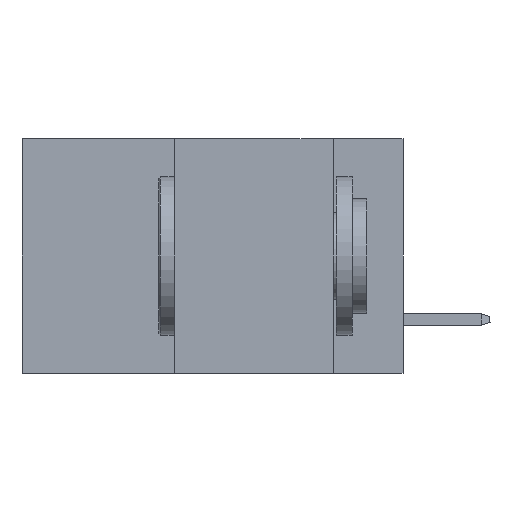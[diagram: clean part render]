
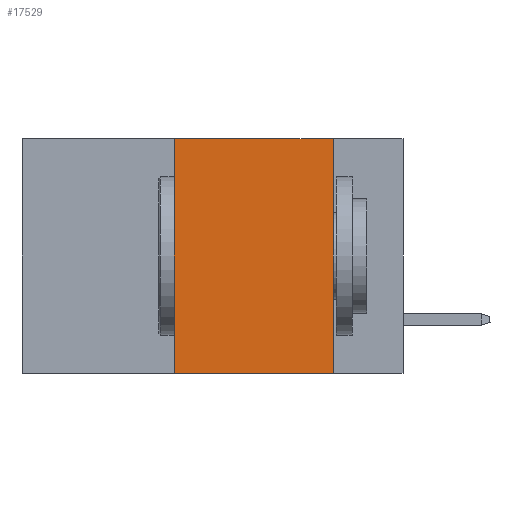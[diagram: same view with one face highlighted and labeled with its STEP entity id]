
A CAD part, left-side view. The second image highlights one B-rep face of the part: STEP entity #17529.
In plain terms, the highlighted planar face has unit normal (-1, 0, 0).
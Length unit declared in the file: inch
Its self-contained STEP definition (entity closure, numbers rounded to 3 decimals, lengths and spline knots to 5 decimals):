
#500 = CARTESIAN_POINT ( 'NONE',  ( 0., 0.36, 0. ) ) ;
#1064 = CARTESIAN_POINT ( 'NONE',  ( 0., 0.36, 0. ) ) ;
#1244 = VERTEX_POINT ( 'NONE', #500 ) ;
#1454 = LINE ( 'NONE', #10286, #23113 ) ;
#3227 = PLANE ( 'NONE',  #13983 ) ;
#3644 = LINE ( 'NONE', #22301, #14648 ) ;
#3739 = VERTEX_POINT ( 'NONE', #22751 ) ;
#4150 = EDGE_LOOP ( 'NONE', ( #15900, #16268, #22699, #14006 ) ) ;
#5653 = CARTESIAN_POINT ( 'NONE',  ( 0., 0.6, 0. ) ) ;
#6527 = DIRECTION ( 'NONE',  ( 0., -1., 0. ) ) ;
#9186 = DIRECTION ( 'NONE',  ( 0., 0., -1. ) ) ;
#10286 = CARTESIAN_POINT ( 'NONE',  ( 0., 0.11, 0. ) ) ;
#11950 = CARTESIAN_POINT ( 'NONE',  ( 0., 0.36, -0.37 ) ) ;
#13103 = VERTEX_POINT ( 'NONE', #11950 ) ;
#13980 = DIRECTION ( 'NONE',  ( 0., 0., -1. ) ) ;
#13983 = AXIS2_PLACEMENT_3D ( 'NONE', #21688, #33968, #9186 ) ;
#14006 = ORIENTED_EDGE ( 'NONE', *, *, #29547, .T. ) ;
#14639 = VERTEX_POINT ( 'NONE', #29910 ) ;
#14648 = VECTOR ( 'NONE', #6527, 39.37008 ) ;
#14670 = LINE ( 'NONE', #5653, #25847 ) ;
#15602 = EDGE_CURVE ( 'NONE', #3739, #14639, #1454, .T. ) ;
#15900 = ORIENTED_EDGE ( 'NONE', *, *, #15602, .F. ) ;
#16268 = ORIENTED_EDGE ( 'NONE', *, *, #18912, .F. ) ;
#16671 = DIRECTION ( 'NONE',  ( 0., 0., 1. ) ) ;
#17529 = ADVANCED_FACE ( 'NONE', ( #21483 ), #3227, .F. ) ;
#18102 = VECTOR ( 'NONE', #16671, 39.37008 ) ;
#18912 = EDGE_CURVE ( 'NONE', #1244, #3739, #14670, .T. ) ;
#21103 = EDGE_CURVE ( 'NONE', #13103, #1244, #28928, .T. ) ;
#21483 = FACE_OUTER_BOUND ( 'NONE', #4150, .T. ) ;
#21688 = CARTESIAN_POINT ( 'NONE',  ( 0., 0.6, 0. ) ) ;
#22301 = CARTESIAN_POINT ( 'NONE',  ( 0., 0.6, -0.37 ) ) ;
#22699 = ORIENTED_EDGE ( 'NONE', *, *, #21103, .F. ) ;
#22751 = CARTESIAN_POINT ( 'NONE',  ( 0., 0.11, 0. ) ) ;
#23113 = VECTOR ( 'NONE', #13980, 39.37008 ) ;
#25847 = VECTOR ( 'NONE', #40079, 39.37008 ) ;
#28928 = LINE ( 'NONE', #1064, #18102 ) ;
#29547 = EDGE_CURVE ( 'NONE', #13103, #14639, #3644, .T. ) ;
#29910 = CARTESIAN_POINT ( 'NONE',  ( 0., 0.11, -0.37 ) ) ;
#33968 = DIRECTION ( 'NONE',  ( 1., 0., 0. ) ) ;
#40079 = DIRECTION ( 'NONE',  ( 0., -1., 0. ) ) ;
